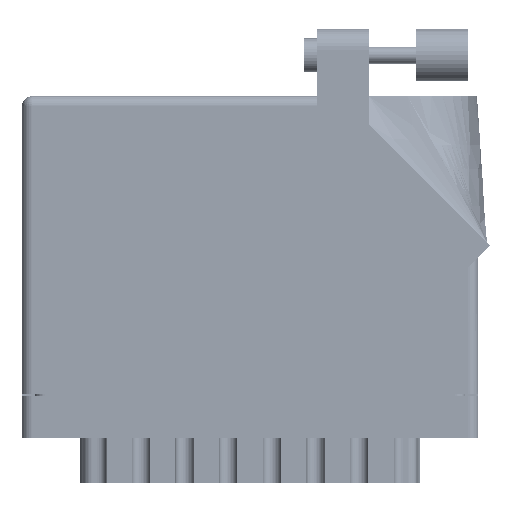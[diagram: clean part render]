
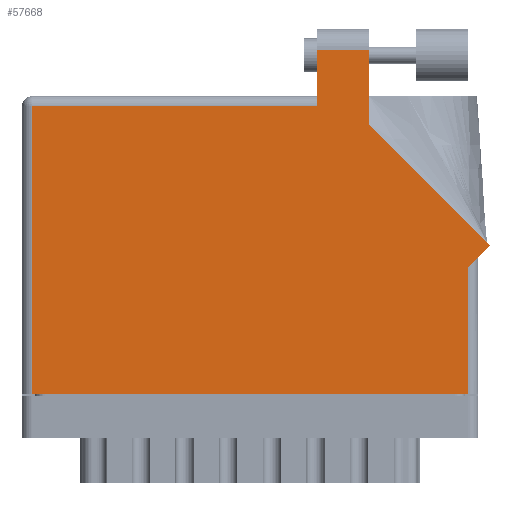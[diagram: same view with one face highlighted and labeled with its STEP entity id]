
A CAD part, front view. The second image highlights one B-rep face of the part: STEP entity #57668.
In plain terms, the highlighted face is planar.
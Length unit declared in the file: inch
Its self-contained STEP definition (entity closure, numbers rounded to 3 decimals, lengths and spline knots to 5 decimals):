
#107 = VERTEX_POINT ( 'NONE', #6924 ) ;
#236 = ORIENTED_EDGE ( 'NONE', *, *, #65034, .T. ) ;
#2418 = DIRECTION ( 'NONE',  ( 0., -1., 0. ) ) ;
#2532 = ORIENTED_EDGE ( 'NONE', *, *, #50473, .T. ) ;
#3473 = VECTOR ( 'NONE', #28685, 39.37008 ) ;
#4536 = ORIENTED_EDGE ( 'NONE', *, *, #71619, .T. ) ;
#5076 = CARTESIAN_POINT ( 'NONE',  ( 2.78871, 0.88571, 0. ) ) ;
#5557 = CARTESIAN_POINT ( 'NONE',  ( 1.758, 2.05, 0. ) ) ;
#6924 = CARTESIAN_POINT ( 'NONE',  ( 2.656, 0., 0. ) ) ;
#7586 = ORIENTED_EDGE ( 'NONE', *, *, #47859, .T. ) ;
#8579 = CARTESIAN_POINT ( 'NONE',  ( 2.78871, 0.88571, 0. ) ) ;
#9304 = LINE ( 'NONE', #68740, #18973 ) ;
#10182 = CARTESIAN_POINT ( 'NONE',  ( 1.758, 1.775, 0. ) ) ;
#13488 = VECTOR ( 'NONE', #19903, 39.37008 ) ;
#13970 = ORIENTED_EDGE ( 'NONE', *, *, #61367, .T. ) ;
#14282 = CARTESIAN_POINT ( 'NONE',  ( 0., 0., 0. ) ) ;
#14965 = VERTEX_POINT ( 'NONE', #5076 ) ;
#16116 = CARTESIAN_POINT ( 'NONE',  ( 2.065, 1.60942, 0. ) ) ;
#16788 = VECTOR ( 'NONE', #61888, 39.37008 ) ;
#18917 = DIRECTION ( 'NONE',  ( 0., 0., -1. ) ) ;
#18956 = DIRECTION ( 'NONE',  ( -1., 0., 0. ) ) ;
#18973 = VECTOR ( 'NONE', #29105, 39.37008 ) ;
#19903 = DIRECTION ( 'NONE',  ( -0.707, 0.707, 0. ) ) ;
#20351 = VERTEX_POINT ( 'NONE', #50842 ) ;
#20412 = VECTOR ( 'NONE', #18956, 39.37008 ) ;
#20687 = VECTOR ( 'NONE', #2418, 39.37008 ) ;
#20791 = ORIENTED_EDGE ( 'NONE', *, *, #40476, .T. ) ;
#22461 = LINE ( 'NONE', #31988, #20687 ) ;
#24607 = DIRECTION ( 'NONE',  ( -1., 0., 0. ) ) ;
#25508 = VECTOR ( 'NONE', #32632, 39.37008 ) ;
#26163 = CARTESIAN_POINT ( 'NONE',  ( 2.065, 1.60942, 0. ) ) ;
#26858 = VERTEX_POINT ( 'NONE', #63607 ) ;
#27174 = DIRECTION ( 'NONE',  ( 0., 1., 0. ) ) ;
#27378 = VERTEX_POINT ( 'NONE', #68411 ) ;
#27687 = FACE_OUTER_BOUND ( 'NONE', #56161, .T. ) ;
#28685 = DIRECTION ( 'NONE',  ( -1., 0., 0. ) ) ;
#29105 = DIRECTION ( 'NONE',  ( 0., 1., 0. ) ) ;
#30033 = ORIENTED_EDGE ( 'NONE', *, *, #71582, .T. ) ;
#30551 = EDGE_CURVE ( 'NONE', #27378, #14965, #57336, .T. ) ;
#30576 = CARTESIAN_POINT ( 'NONE',  ( 2.065, 2.05, 0. ) ) ;
#31988 = CARTESIAN_POINT ( 'NONE',  ( 0.062, 0., 0. ) ) ;
#32597 = LINE ( 'NONE', #16116, #51981 ) ;
#32632 = DIRECTION ( 'NONE',  ( 0., -1., 0. ) ) ;
#33391 = EDGE_CURVE ( 'NONE', #107, #27378, #9304, .T. ) ;
#35425 = LINE ( 'NONE', #47093, #20412 ) ;
#35660 = AXIS2_PLACEMENT_3D ( 'NONE', #46573, #18917, #24607 ) ;
#36599 = VERTEX_POINT ( 'NONE', #30576 ) ;
#37823 = VERTEX_POINT ( 'NONE', #47967 ) ;
#40309 = CARTESIAN_POINT ( 'NONE',  ( 0.062, 1.713, 0. ) ) ;
#40476 = EDGE_CURVE ( 'NONE', #14965, #50947, #68100, .T. ) ;
#40891 = PLANE ( 'NONE',  #35660 ) ;
#42611 = DIRECTION ( 'NONE',  ( 1., 0., 0. ) ) ;
#46573 = CARTESIAN_POINT ( 'NONE',  ( 0., 1.775, 0. ) ) ;
#47093 = CARTESIAN_POINT ( 'NONE',  ( 0., 1.713, 0. ) ) ;
#47859 = EDGE_CURVE ( 'NONE', #20351, #107, #68460, .T. ) ;
#47967 = CARTESIAN_POINT ( 'NONE',  ( 1.758, 2.05, 0. ) ) ;
#49291 = VERTEX_POINT ( 'NONE', #40309 ) ;
#50473 = EDGE_CURVE ( 'NONE', #36599, #37823, #56363, .T. ) ;
#50842 = CARTESIAN_POINT ( 'NONE',  ( 0.062, 0., 0. ) ) ;
#50947 = VERTEX_POINT ( 'NONE', #26163 ) ;
#51981 = VECTOR ( 'NONE', #27174, 39.37008 ) ;
#56161 = EDGE_LOOP ( 'NONE', ( #30033, #2532, #4536, #13970, #236, #7586, #60347, #63431, #20791 ) ) ;
#56363 = LINE ( 'NONE', #5557, #3473 ) ;
#57336 = LINE ( 'NONE', #67766, #16788 ) ;
#57668 = ADVANCED_FACE ( 'NONE', ( #27687 ), #40891, .F. ) ;
#60347 = ORIENTED_EDGE ( 'NONE', *, *, #33391, .T. ) ;
#60592 = VECTOR ( 'NONE', #42611, 39.37008 ) ;
#61367 = EDGE_CURVE ( 'NONE', #26858, #49291, #35425, .T. ) ;
#61888 = DIRECTION ( 'NONE',  ( 0.707, 0.707, 0. ) ) ;
#63431 = ORIENTED_EDGE ( 'NONE', *, *, #30551, .T. ) ;
#63607 = CARTESIAN_POINT ( 'NONE',  ( 1.758, 1.713, 0. ) ) ;
#65034 = EDGE_CURVE ( 'NONE', #49291, #20351, #22461, .T. ) ;
#65180 = LINE ( 'NONE', #10182, #25508 ) ;
#67766 = CARTESIAN_POINT ( 'NONE',  ( 2.718, 0.815, 0. ) ) ;
#68100 = LINE ( 'NONE', #8579, #13488 ) ;
#68411 = CARTESIAN_POINT ( 'NONE',  ( 2.656, 0.753, 0. ) ) ;
#68460 = LINE ( 'NONE', #14282, #60592 ) ;
#68740 = CARTESIAN_POINT ( 'NONE',  ( 2.656, 0.815, 0. ) ) ;
#71582 = EDGE_CURVE ( 'NONE', #50947, #36599, #32597, .T. ) ;
#71619 = EDGE_CURVE ( 'NONE', #37823, #26858, #65180, .T. ) ;
